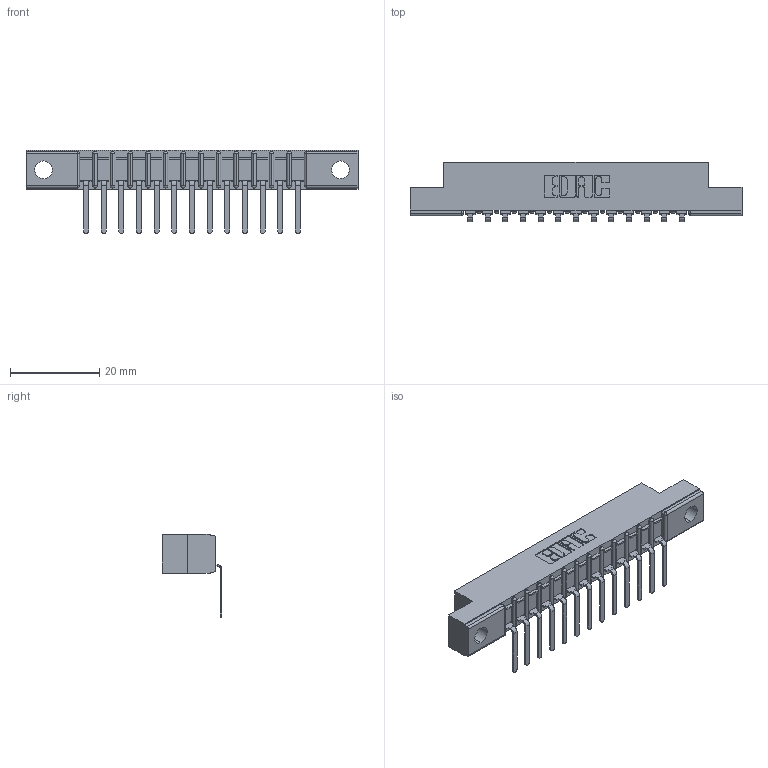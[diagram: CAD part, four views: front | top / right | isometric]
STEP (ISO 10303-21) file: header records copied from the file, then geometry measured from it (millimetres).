
FILE_DESCRIPTION (( 'STEP AP203' ), '1' );
FILE_NAME ('307-013-457-104.STEP', '2020-09-25T14:20:34', ( '' ), ( '' ), 'SwSTEP 2.0', 'SolidWorks 2020', '' );
FILE_SCHEMA (( 'CONFIG_CONTROL_DESIGN' ));
Length unit declared in the file: inch
Products named in the file (6): 307 Part_.156 Dia Mounting Holes; 307-013-457-104; 307-290-002_557; 345-250-001_345-250-005-103; #2516; #34854
Assembly tree (59 placements, depth 2):
  307-013-457-104
    307 Part_.156 Dia Mounting Holes
    307-290-002_557  x13
  #34854
    #25402
    #2516  x42
    345-250-001_345-250-005-103  x2
Bounding box: 74.52 x 13.32 x 18.67 mm (x, y, z)
Volume: 4844.3 mm3; surface area: 8415.7 mm2
Topology: 14 solids, 14 shells, 1160 faces, 3531 edges, 2314 vertices
Faces by surface type: plane 695, cylinder 437, sphere 28
Entity records: 33228 total; most frequent: CARTESIAN_POINT 5583, ORIENTED_EDGE 5554, DIRECTION 5469, EDGE_CURVE 2776, VECTOR 2137, LINE 2113, VERTEX_POINT 1806, AXIS2_PLACEMENT_3D 1639
